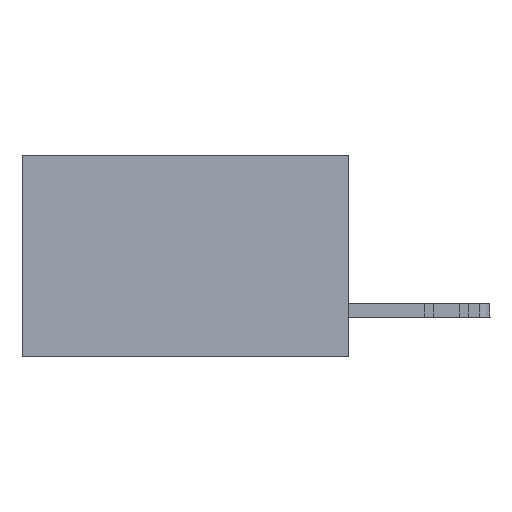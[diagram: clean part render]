
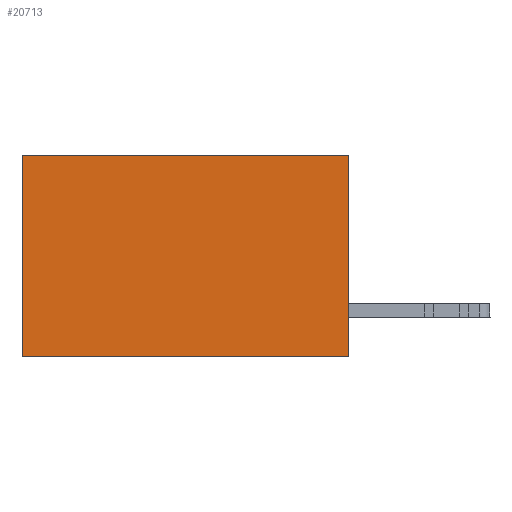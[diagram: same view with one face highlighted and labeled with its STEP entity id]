
A CAD part, left-side view. The second image highlights one B-rep face of the part: STEP entity #20713.
In plain terms, the highlighted planar face has unit normal (-1, 0, 0).
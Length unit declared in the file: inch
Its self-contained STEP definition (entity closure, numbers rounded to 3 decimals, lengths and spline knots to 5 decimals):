
#1323 = ORIENTED_EDGE ( 'NONE', *, *, #15979, .F. ) ;
#1884 = FACE_OUTER_BOUND ( 'NONE', #26503, .T. ) ;
#3474 = VERTEX_POINT ( 'NONE', #7016 ) ;
#4116 = VERTEX_POINT ( 'NONE', #11163 ) ;
#4537 = DIRECTION ( 'NONE',  ( 1., 0., 0. ) ) ;
#4776 = LINE ( 'NONE', #5401, #16067 ) ;
#5401 = CARTESIAN_POINT ( 'NONE',  ( 0.298, 0., -0.37 ) ) ;
#7016 = CARTESIAN_POINT ( 'NONE',  ( 0.298, 0., -0.37 ) ) ;
#8212 = DIRECTION ( 'NONE',  ( 0., 1., 0. ) ) ;
#9551 = VECTOR ( 'NONE', #8212, 39.37008 ) ;
#9932 = AXIS2_PLACEMENT_3D ( 'NONE', #11238, #4537, #20298 ) ;
#11163 = CARTESIAN_POINT ( 'NONE',  ( 0.298, 0.6, 0. ) ) ;
#11238 = CARTESIAN_POINT ( 'NONE',  ( 0.298, 0., 0. ) ) ;
#11974 = DIRECTION ( 'NONE',  ( 0., 0., -1. ) ) ;
#14367 = DIRECTION ( 'NONE',  ( 0., 0., -1. ) ) ;
#14506 = ORIENTED_EDGE ( 'NONE', *, *, #24865, .F. ) ;
#15979 = EDGE_CURVE ( 'NONE', #17949, #3474, #16501, .T. ) ;
#16067 = VECTOR ( 'NONE', #25426, 39.37008 ) ;
#16501 = LINE ( 'NONE', #18833, #27542 ) ;
#16766 = VECTOR ( 'NONE', #11974, 39.37008 ) ;
#17897 = CARTESIAN_POINT ( 'NONE',  ( 0.298, 0.6, -0.37 ) ) ;
#17949 = VERTEX_POINT ( 'NONE', #19852 ) ;
#18046 = PLANE ( 'NONE',  #9932 ) ;
#18814 = CARTESIAN_POINT ( 'NONE',  ( 0.298, 0.6, 0. ) ) ;
#18833 = CARTESIAN_POINT ( 'NONE',  ( 0.298, 0., 0. ) ) ;
#19852 = CARTESIAN_POINT ( 'NONE',  ( 0.298, 0., 0. ) ) ;
#20298 = DIRECTION ( 'NONE',  ( 0., 0., -1. ) ) ;
#20713 = ADVANCED_FACE ( 'NONE', ( #1884 ), #18046, .F. ) ;
#20871 = ORIENTED_EDGE ( 'NONE', *, *, #22474, .T. ) ;
#21949 = VERTEX_POINT ( 'NONE', #17897 ) ;
#22474 = EDGE_CURVE ( 'NONE', #17949, #4116, #27274, .T. ) ;
#22683 = LINE ( 'NONE', #18814, #16766 ) ;
#24232 = ORIENTED_EDGE ( 'NONE', *, *, #24836, .T. ) ;
#24836 = EDGE_CURVE ( 'NONE', #4116, #21949, #22683, .T. ) ;
#24865 = EDGE_CURVE ( 'NONE', #3474, #21949, #4776, .T. ) ;
#25426 = DIRECTION ( 'NONE',  ( 0., 1., 0. ) ) ;
#26123 = CARTESIAN_POINT ( 'NONE',  ( 0.298, 0., 0. ) ) ;
#26503 = EDGE_LOOP ( 'NONE', ( #24232, #14506, #1323, #20871 ) ) ;
#27274 = LINE ( 'NONE', #26123, #9551 ) ;
#27542 = VECTOR ( 'NONE', #14367, 39.37008 ) ;
